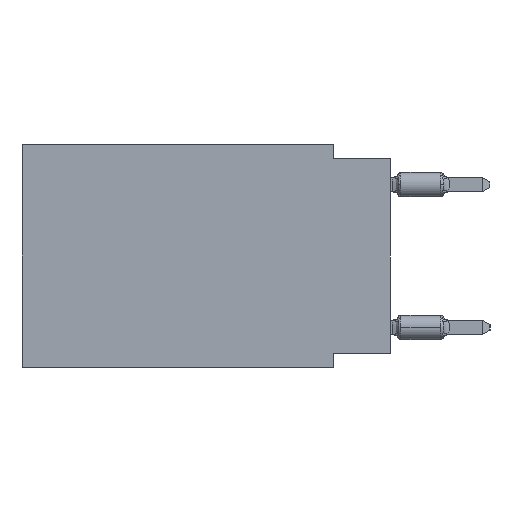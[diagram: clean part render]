
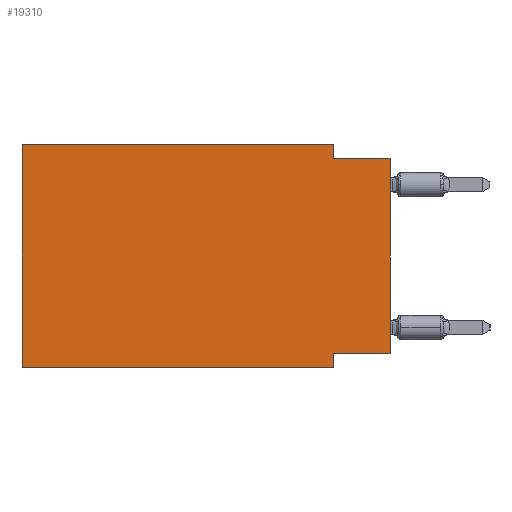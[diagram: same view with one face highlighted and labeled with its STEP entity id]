
A CAD part, left-side view. The second image highlights one B-rep face of the part: STEP entity #19310.
In plain terms, the highlighted planar face has unit normal (-1, 0, 0).
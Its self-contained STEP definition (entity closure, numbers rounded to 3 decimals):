
#196 = DIRECTION ( 'NONE',  ( 0., 0., 1. ) ) ;
#207 = EDGE_CURVE ( 'NONE', #41385, #32744, #4252, .T. ) ;
#2868 = EDGE_CURVE ( 'NONE', #32744, #51190, #24020, .T. ) ;
#4252 = LINE ( 'NONE', #31531, #34204 ) ;
#4318 = VERTEX_POINT ( 'NONE', #40170 ) ;
#4392 = CARTESIAN_POINT ( 'NONE',  ( 0., 16.383, 0. ) ) ;
#6865 = EDGE_CURVE ( 'NONE', #9810, #4318, #54431, .T. ) ;
#8809 = DIRECTION ( 'NONE',  ( 0., 0., 1. ) ) ;
#9127 = ORIENTED_EDGE ( 'NONE', *, *, #55166, .T. ) ;
#9648 = DIRECTION ( 'NONE',  ( 0., 0., -1. ) ) ;
#9810 = VERTEX_POINT ( 'NONE', #23139 ) ;
#14074 = ORIENTED_EDGE ( 'NONE', *, *, #6865, .F. ) ;
#15336 = CARTESIAN_POINT ( 'NONE',  ( 0., 16.383, -9.906 ) ) ;
#15775 = DIRECTION ( 'NONE',  ( 1., 0., 0. ) ) ;
#15821 = VERTEX_POINT ( 'NONE', #18668 ) ;
#15853 = LINE ( 'NONE', #39546, #20703 ) ;
#16186 = CARTESIAN_POINT ( 'NONE',  ( 0., 0., -9.271 ) ) ;
#18344 = VECTOR ( 'NONE', #42494, 1000. ) ;
#18668 = CARTESIAN_POINT ( 'NONE',  ( 0., 2.54, 0. ) ) ;
#19310 = ADVANCED_FACE ( 'NONE', ( #33783 ), #30465, .F. ) ;
#20508 = VERTEX_POINT ( 'NONE', #28758 ) ;
#20576 = ORIENTED_EDGE ( 'NONE', *, *, #38927, .F. ) ;
#20589 = CARTESIAN_POINT ( 'NONE',  ( 0., 2.54, 0. ) ) ;
#20703 = VECTOR ( 'NONE', #57804, 1000. ) ;
#20959 = VECTOR ( 'NONE', #9648, 1000. ) ;
#22226 = EDGE_CURVE ( 'NONE', #15821, #20508, #33801, .T. ) ;
#22592 = VERTEX_POINT ( 'NONE', #23844 ) ;
#23139 = CARTESIAN_POINT ( 'NONE',  ( 0., 16.383, -9.906 ) ) ;
#23430 = CARTESIAN_POINT ( 'NONE',  ( 0., 2.54, -9.906 ) ) ;
#23844 = CARTESIAN_POINT ( 'NONE',  ( 0., 0., -0.635 ) ) ;
#24020 = LINE ( 'NONE', #23430, #20959 ) ;
#24291 = DIRECTION ( 'NONE',  ( 0., -1., 0. ) ) ;
#24392 = EDGE_CURVE ( 'NONE', #9810, #51190, #32445, .T. ) ;
#27031 = DIRECTION ( 'NONE',  ( 0., 1., 0. ) ) ;
#28758 = CARTESIAN_POINT ( 'NONE',  ( 0., 2.54, -0.635 ) ) ;
#30465 = PLANE ( 'NONE',  #34308 ) ;
#30784 = ORIENTED_EDGE ( 'NONE', *, *, #22226, .F. ) ;
#31531 = CARTESIAN_POINT ( 'NONE',  ( 0., 0., -9.271 ) ) ;
#32445 = LINE ( 'NONE', #15336, #46718 ) ;
#32744 = VERTEX_POINT ( 'NONE', #58245 ) ;
#33783 = FACE_OUTER_BOUND ( 'NONE', #59008, .T. ) ;
#33801 = LINE ( 'NONE', #20589, #18344 ) ;
#34197 = ORIENTED_EDGE ( 'NONE', *, *, #47488, .F. ) ;
#34204 = VECTOR ( 'NONE', #27031, 1000. ) ;
#34308 = AXIS2_PLACEMENT_3D ( 'NONE', #48744, #15775, #56529 ) ;
#36625 = VECTOR ( 'NONE', #196, 1000. ) ;
#38798 = ORIENTED_EDGE ( 'NONE', *, *, #2868, .F. ) ;
#38927 = EDGE_CURVE ( 'NONE', #20508, #22592, #15853, .T. ) ;
#39546 = CARTESIAN_POINT ( 'NONE',  ( 0., 0., -0.635 ) ) ;
#40170 = CARTESIAN_POINT ( 'NONE',  ( 0., 16.383, 0. ) ) ;
#41385 = VERTEX_POINT ( 'NONE', #16186 ) ;
#42494 = DIRECTION ( 'NONE',  ( 0., 0., -1. ) ) ;
#43988 = ORIENTED_EDGE ( 'NONE', *, *, #24392, .T. ) ;
#46198 = CARTESIAN_POINT ( 'NONE',  ( 0., 2.54, -9.906 ) ) ;
#46718 = VECTOR ( 'NONE', #47109, 1000. ) ;
#47060 = CARTESIAN_POINT ( 'NONE',  ( 0., 16.383, 0. ) ) ;
#47109 = DIRECTION ( 'NONE',  ( 0., -1., 0. ) ) ;
#47362 = LINE ( 'NONE', #47060, #55684 ) ;
#47488 = EDGE_CURVE ( 'NONE', #4318, #15821, #47362, .T. ) ;
#48744 = CARTESIAN_POINT ( 'NONE',  ( 0., 16.383, 0. ) ) ;
#49265 = CARTESIAN_POINT ( 'NONE',  ( 0., 0., 0. ) ) ;
#51190 = VERTEX_POINT ( 'NONE', #46198 ) ;
#53940 = ORIENTED_EDGE ( 'NONE', *, *, #207, .F. ) ;
#54431 = LINE ( 'NONE', #4392, #36625 ) ;
#55166 = EDGE_CURVE ( 'NONE', #41385, #22592, #58248, .T. ) ;
#55684 = VECTOR ( 'NONE', #24291, 1000. ) ;
#56529 = DIRECTION ( 'NONE',  ( 0., 0., -1. ) ) ;
#57804 = DIRECTION ( 'NONE',  ( 0., -1., 0. ) ) ;
#58245 = CARTESIAN_POINT ( 'NONE',  ( 0., 2.54, -9.271 ) ) ;
#58248 = LINE ( 'NONE', #49265, #58657 ) ;
#58657 = VECTOR ( 'NONE', #8809, 1000. ) ;
#59008 = EDGE_LOOP ( 'NONE', ( #9127, #20576, #30784, #34197, #14074, #43988, #38798, #53940 ) ) ;
